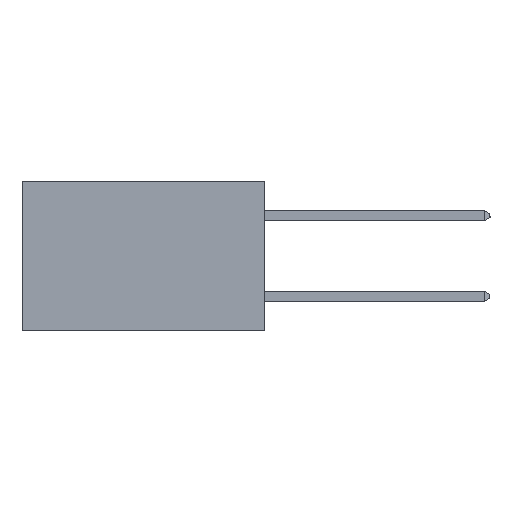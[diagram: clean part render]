
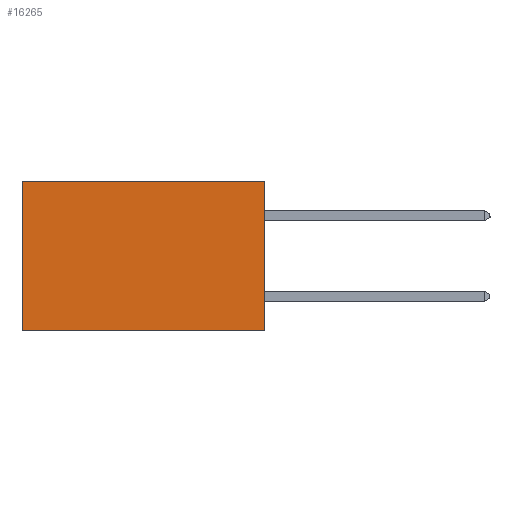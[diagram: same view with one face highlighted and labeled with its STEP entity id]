
A CAD part, left-side view. The second image highlights one B-rep face of the part: STEP entity #16265.
In plain terms, the highlighted planar face has unit normal (-1, 0, 0).
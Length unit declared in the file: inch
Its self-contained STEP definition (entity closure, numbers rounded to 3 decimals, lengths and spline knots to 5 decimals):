
#638 = VERTEX_POINT ( 'NONE', #6434 ) ;
#807 = EDGE_LOOP ( 'NONE', ( #7896, #11807, #14629, #10776 ) ) ;
#1021 = AXIS2_PLACEMENT_3D ( 'NONE', #6566, #17321, #8082 ) ;
#1771 = LINE ( 'NONE', #4107, #13682 ) ;
#2032 = CARTESIAN_POINT ( 'NONE',  ( 0.298, 0., 0. ) ) ;
#2080 = EDGE_CURVE ( 'NONE', #638, #7570, #8007, .T. ) ;
#3326 = CARTESIAN_POINT ( 'NONE',  ( 0.298, 0., -0.37 ) ) ;
#3865 = VECTOR ( 'NONE', #17230, 39.37008 ) ;
#4107 = CARTESIAN_POINT ( 'NONE',  ( 0.298, 0.6, 0. ) ) ;
#4307 = LINE ( 'NONE', #2032, #12041 ) ;
#4924 = DIRECTION ( 'NONE',  ( 0., 1., 0. ) ) ;
#5694 = DIRECTION ( 'NONE',  ( 0., 0., -1. ) ) ;
#6434 = CARTESIAN_POINT ( 'NONE',  ( 0.298, 0., 0. ) ) ;
#6566 = CARTESIAN_POINT ( 'NONE',  ( 0.298, 0., 0. ) ) ;
#7570 = VERTEX_POINT ( 'NONE', #8400 ) ;
#7896 = ORIENTED_EDGE ( 'NONE', *, *, #11077, .T. ) ;
#8007 = LINE ( 'NONE', #14051, #3865 ) ;
#8082 = DIRECTION ( 'NONE',  ( 0., 0., -1. ) ) ;
#8189 = VERTEX_POINT ( 'NONE', #11179 ) ;
#8243 = DIRECTION ( 'NONE',  ( 0., 1., 0. ) ) ;
#8400 = CARTESIAN_POINT ( 'NONE',  ( 0.298, 0., -0.37 ) ) ;
#9123 = FACE_OUTER_BOUND ( 'NONE', #807, .T. ) ;
#10776 = ORIENTED_EDGE ( 'NONE', *, *, #15650, .T. ) ;
#11077 = EDGE_CURVE ( 'NONE', #8189, #17577, #1771, .T. ) ;
#11179 = CARTESIAN_POINT ( 'NONE',  ( 0.298, 0.6, 0. ) ) ;
#11428 = EDGE_CURVE ( 'NONE', #7570, #17577, #16102, .T. ) ;
#11807 = ORIENTED_EDGE ( 'NONE', *, *, #11428, .F. ) ;
#11960 = VECTOR ( 'NONE', #4924, 39.37008 ) ;
#12041 = VECTOR ( 'NONE', #8243, 39.37008 ) ;
#13682 = VECTOR ( 'NONE', #5694, 39.37008 ) ;
#14051 = CARTESIAN_POINT ( 'NONE',  ( 0.298, 0., 0. ) ) ;
#14629 = ORIENTED_EDGE ( 'NONE', *, *, #2080, .F. ) ;
#15388 = CARTESIAN_POINT ( 'NONE',  ( 0.298, 0.6, -0.37 ) ) ;
#15650 = EDGE_CURVE ( 'NONE', #638, #8189, #4307, .T. ) ;
#16102 = LINE ( 'NONE', #3326, #11960 ) ;
#16265 = ADVANCED_FACE ( 'NONE', ( #9123 ), #17258, .F. ) ;
#17230 = DIRECTION ( 'NONE',  ( 0., 0., -1. ) ) ;
#17258 = PLANE ( 'NONE',  #1021 ) ;
#17321 = DIRECTION ( 'NONE',  ( 1., 0., 0. ) ) ;
#17577 = VERTEX_POINT ( 'NONE', #15388 ) ;
